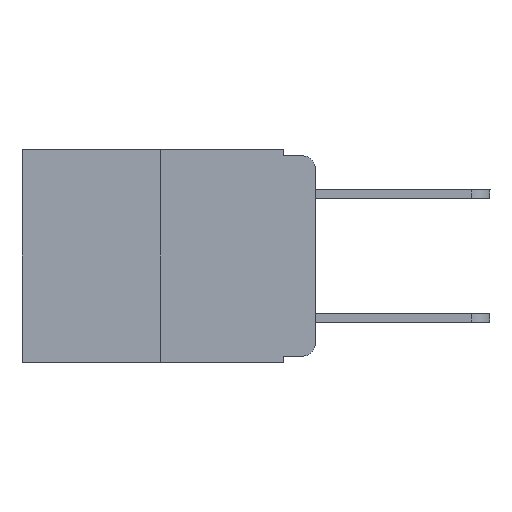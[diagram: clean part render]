
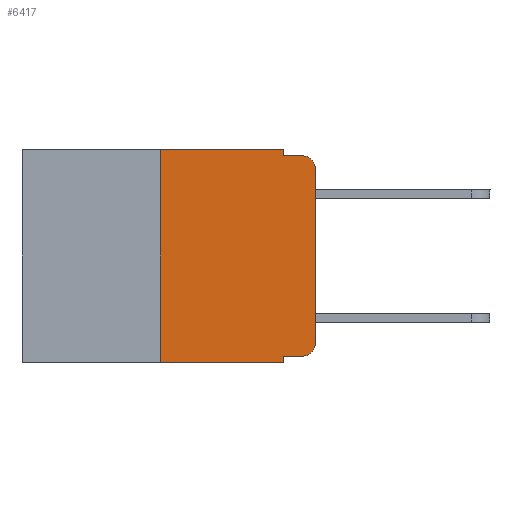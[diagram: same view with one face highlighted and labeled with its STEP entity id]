
A CAD part, left-side view. The second image highlights one B-rep face of the part: STEP entity #6417.
In plain terms, the highlighted planar face has unit normal (-1, 0, 0).
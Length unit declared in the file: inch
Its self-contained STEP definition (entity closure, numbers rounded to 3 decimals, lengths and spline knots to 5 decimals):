
#188 = EDGE_CURVE ( 'NONE', #4973, #3182, #6538, .T. ) ;
#526 = DIRECTION ( 'NONE',  ( 0., -1., 0. ) ) ;
#571 = DIRECTION ( 'NONE',  ( -1., 0., 0. ) ) ;
#624 = VERTEX_POINT ( 'NONE', #12418 ) ;
#672 = CARTESIAN_POINT ( 'NONE',  ( 0., 0.02, -0.313 ) ) ;
#832 = EDGE_LOOP ( 'NONE', ( #7410, #10279, #8010, #8024, #3669, #11857, #11531, #11722, #11051, #1362 ) ) ;
#1098 = EDGE_CURVE ( 'NONE', #624, #8898, #4123, .T. ) ;
#1362 = ORIENTED_EDGE ( 'NONE', *, *, #1098, .T. ) ;
#1431 = EDGE_CURVE ( 'NONE', #10303, #4570, #8902, .T. ) ;
#1444 = DIRECTION ( 'NONE',  ( 0., 0., 1. ) ) ;
#1609 = EDGE_CURVE ( 'NONE', #4570, #3069, #10253, .T. ) ;
#1626 = EDGE_CURVE ( 'NONE', #9839, #3182, #6260, .T. ) ;
#1737 = CARTESIAN_POINT ( 'NONE',  ( 0., 0.051, 0. ) ) ;
#2051 = CARTESIAN_POINT ( 'NONE',  ( 0., 0.051, -0.333 ) ) ;
#2063 = AXIS2_PLACEMENT_3D ( 'NONE', #7664, #7874, #11120 ) ;
#2331 = VECTOR ( 'NONE', #11554, 39.37008 ) ;
#2339 = VECTOR ( 'NONE', #6105, 39.37008 ) ;
#3069 = VERTEX_POINT ( 'NONE', #1737 ) ;
#3079 = CARTESIAN_POINT ( 'NONE',  ( 0., 0.051, -0.343 ) ) ;
#3182 = VERTEX_POINT ( 'NONE', #13648 ) ;
#3258 = CARTESIAN_POINT ( 'NONE',  ( 0., 0.473, -0.343 ) ) ;
#3447 = VECTOR ( 'NONE', #7608, 39.37008 ) ;
#3452 = CARTESIAN_POINT ( 'NONE',  ( 0., 0.25, -0.343 ) ) ;
#3669 = ORIENTED_EDGE ( 'NONE', *, *, #1609, .F. ) ;
#3824 = LINE ( 'NONE', #11474, #2339 ) ;
#4056 = LINE ( 'NONE', #8258, #6708 ) ;
#4123 = CIRCLE ( 'NONE', #5969, 0.02 ) ;
#4257 = LINE ( 'NONE', #3258, #3447 ) ;
#4313 = VECTOR ( 'NONE', #1444, 39.37008 ) ;
#4570 = VERTEX_POINT ( 'NONE', #8600 ) ;
#4907 = LINE ( 'NONE', #7243, #2331 ) ;
#4973 = VERTEX_POINT ( 'NONE', #11570 ) ;
#5072 = DIRECTION ( 'NONE',  ( -1., 0., 0. ) ) ;
#5303 = LINE ( 'NONE', #10775, #8884 ) ;
#5868 = AXIS2_PLACEMENT_3D ( 'NONE', #13555, #571, #9507 ) ;
#5969 = AXIS2_PLACEMENT_3D ( 'NONE', #672, #5072, #10197 ) ;
#6105 = DIRECTION ( 'NONE',  ( 0., 0., -1. ) ) ;
#6249 = EDGE_CURVE ( 'NONE', #8898, #4973, #5303, .T. ) ;
#6260 = LINE ( 'NONE', #12632, #9037 ) ;
#6320 = DIRECTION ( 'NONE',  ( 0., 0., 1. ) ) ;
#6417 = ADVANCED_FACE ( 'NONE', ( #9858 ), #8788, .F. ) ;
#6538 = CIRCLE ( 'NONE', #5868, 0.02 ) ;
#6641 = CARTESIAN_POINT ( 'NONE',  ( 0., 0.25, 0. ) ) ;
#6708 = VECTOR ( 'NONE', #8384, 39.37008 ) ;
#7018 = VERTEX_POINT ( 'NONE', #2051 ) ;
#7091 = EDGE_CURVE ( 'NONE', #10303, #10498, #4257, .T. ) ;
#7224 = VECTOR ( 'NONE', #526, 39.37008 ) ;
#7243 = CARTESIAN_POINT ( 'NONE',  ( 0., 0.051, 0. ) ) ;
#7378 = EDGE_CURVE ( 'NONE', #7018, #10498, #4907, .T. ) ;
#7410 = ORIENTED_EDGE ( 'NONE', *, *, #6249, .T. ) ;
#7608 = DIRECTION ( 'NONE',  ( 0., -1., 0. ) ) ;
#7664 = CARTESIAN_POINT ( 'NONE',  ( 0., 0.473, 0. ) ) ;
#7874 = DIRECTION ( 'NONE',  ( 1., 0., 0. ) ) ;
#7887 = EDGE_CURVE ( 'NONE', #3069, #9839, #3824, .T. ) ;
#8010 = ORIENTED_EDGE ( 'NONE', *, *, #1626, .F. ) ;
#8024 = ORIENTED_EDGE ( 'NONE', *, *, #7887, .F. ) ;
#8258 = CARTESIAN_POINT ( 'NONE',  ( 0., 0.051, -0.333 ) ) ;
#8384 = DIRECTION ( 'NONE',  ( 0., -1., 0. ) ) ;
#8600 = CARTESIAN_POINT ( 'NONE',  ( 0., 0.25, 0. ) ) ;
#8788 = PLANE ( 'NONE',  #2063 ) ;
#8884 = VECTOR ( 'NONE', #6320, 39.37008 ) ;
#8898 = VERTEX_POINT ( 'NONE', #13778 ) ;
#8902 = LINE ( 'NONE', #6641, #4313 ) ;
#8908 = EDGE_CURVE ( 'NONE', #7018, #624, #4056, .T. ) ;
#9037 = VECTOR ( 'NONE', #13892, 39.37008 ) ;
#9507 = DIRECTION ( 'NONE',  ( 0., 0., -1. ) ) ;
#9839 = VERTEX_POINT ( 'NONE', #13233 ) ;
#9858 = FACE_OUTER_BOUND ( 'NONE', #832, .T. ) ;
#10197 = DIRECTION ( 'NONE',  ( 0., 0., -1. ) ) ;
#10253 = LINE ( 'NONE', #12769, #7224 ) ;
#10279 = ORIENTED_EDGE ( 'NONE', *, *, #188, .T. ) ;
#10303 = VERTEX_POINT ( 'NONE', #3452 ) ;
#10498 = VERTEX_POINT ( 'NONE', #3079 ) ;
#10775 = CARTESIAN_POINT ( 'NONE',  ( 0., 0., 0. ) ) ;
#11051 = ORIENTED_EDGE ( 'NONE', *, *, #8908, .T. ) ;
#11120 = DIRECTION ( 'NONE',  ( 0., 0., -1. ) ) ;
#11474 = CARTESIAN_POINT ( 'NONE',  ( 0., 0.051, 0. ) ) ;
#11531 = ORIENTED_EDGE ( 'NONE', *, *, #7091, .T. ) ;
#11554 = DIRECTION ( 'NONE',  ( 0., 0., -1. ) ) ;
#11570 = CARTESIAN_POINT ( 'NONE',  ( 0., 0., -0.03 ) ) ;
#11722 = ORIENTED_EDGE ( 'NONE', *, *, #7378, .F. ) ;
#11857 = ORIENTED_EDGE ( 'NONE', *, *, #1431, .F. ) ;
#12418 = CARTESIAN_POINT ( 'NONE',  ( 0., 0.02, -0.333 ) ) ;
#12632 = CARTESIAN_POINT ( 'NONE',  ( 0., 0.051, -0.01 ) ) ;
#12769 = CARTESIAN_POINT ( 'NONE',  ( 0., 0.473, 0. ) ) ;
#13233 = CARTESIAN_POINT ( 'NONE',  ( 0., 0.051, -0.01 ) ) ;
#13555 = CARTESIAN_POINT ( 'NONE',  ( 0., 0.02, -0.03 ) ) ;
#13648 = CARTESIAN_POINT ( 'NONE',  ( 0., 0.02, -0.01 ) ) ;
#13778 = CARTESIAN_POINT ( 'NONE',  ( 0., 0., -0.313 ) ) ;
#13892 = DIRECTION ( 'NONE',  ( 0., -1., 0. ) ) ;
